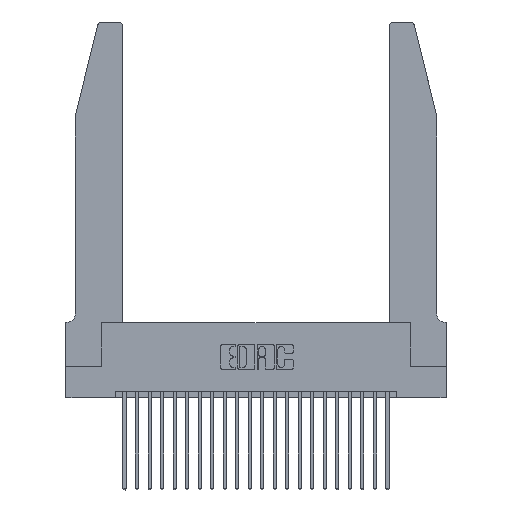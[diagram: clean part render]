
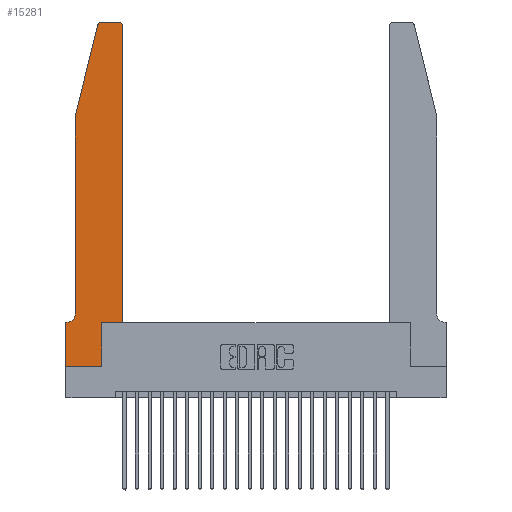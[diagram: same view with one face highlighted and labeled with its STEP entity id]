
A CAD part, top view. The second image highlights one B-rep face of the part: STEP entity #15281.
In plain terms, the highlighted planar face has unit normal (0, 0, 1).
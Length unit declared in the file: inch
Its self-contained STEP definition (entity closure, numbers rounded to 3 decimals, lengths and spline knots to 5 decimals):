
#43 = ORIENTED_EDGE ( 'NONE', *, *, #3046, .T. ) ;
#117 = VERTEX_POINT ( 'NONE', #5731 ) ;
#277 = ORIENTED_EDGE ( 'NONE', *, *, #18983, .T. ) ;
#382 = EDGE_LOOP ( 'NONE', ( #22888, #17297, #6636, #10401, #23073, #19586, #23817, #277, #12710, #6812, #18889, #43 ) ) ;
#537 = DIRECTION ( 'NONE',  ( 1., 0., 0. ) ) ;
#560 = LINE ( 'NONE', #15938, #16672 ) ;
#587 = EDGE_CURVE ( 'NONE', #2119, #10231, #1317, .T. ) ;
#693 = DIRECTION ( 'NONE',  ( 0., 0., 1. ) ) ;
#1015 = CARTESIAN_POINT ( 'NONE',  ( 0.0755, 2., 0.37 ) ) ;
#1059 = CARTESIAN_POINT ( 'NONE',  ( 0.0755, 0.42, 0.37 ) ) ;
#1317 = LINE ( 'NONE', #3193, #20154 ) ;
#1462 = VECTOR ( 'NONE', #9100, 39.37008 ) ;
#2029 = EDGE_CURVE ( 'NONE', #117, #14625, #18886, .T. ) ;
#2119 = VERTEX_POINT ( 'NONE', #3431 ) ;
#2405 = CARTESIAN_POINT ( 'NONE',  ( 0.284, 2.75, 0.37 ) ) ;
#2757 = CARTESIAN_POINT ( 'NONE',  ( 0., 0.35, 0.37 ) ) ;
#3012 = CARTESIAN_POINT ( 'NONE',  ( 0., 0., 0.37 ) ) ;
#3046 = EDGE_CURVE ( 'NONE', #17111, #22062, #6576, .T. ) ;
#3119 = VECTOR ( 'NONE', #14447, 39.37008 ) ;
#3193 = CARTESIAN_POINT ( 'NONE',  ( 0.0755, 0.35, 0.37 ) ) ;
#3431 = CARTESIAN_POINT ( 'NONE',  ( 0.0055, 0.35, 0.37 ) ) ;
#3630 = VERTEX_POINT ( 'NONE', #12774 ) ;
#3832 = CARTESIAN_POINT ( 'NONE',  ( 0.0055, 0.42, 0.37 ) ) ;
#3883 = CIRCLE ( 'NONE', #12302, 0.03 ) ;
#4542 = CARTESIAN_POINT ( 'NONE',  ( 0.284, 2.72, 0.37 ) ) ;
#4727 = VERTEX_POINT ( 'NONE', #1059 ) ;
#4865 = DIRECTION ( 'NONE',  ( -0.239, -0.971, 0. ) ) ;
#5518 = LINE ( 'NONE', #23951, #3119 ) ;
#5731 = CARTESIAN_POINT ( 'NONE',  ( 0.25487, 2.72718, 0.37 ) ) ;
#6071 = DIRECTION ( 'NONE',  ( 0., 0., 1. ) ) ;
#6576 = CIRCLE ( 'NONE', #12965, 0.03 ) ;
#6636 = ORIENTED_EDGE ( 'NONE', *, *, #2029, .T. ) ;
#6812 = ORIENTED_EDGE ( 'NONE', *, *, #21663, .T. ) ;
#7202 = CARTESIAN_POINT ( 'NONE',  ( 0.0755, 2., 0.37 ) ) ;
#7475 = EDGE_CURVE ( 'NONE', #14667, #3630, #17307, .T. ) ;
#7764 = CARTESIAN_POINT ( 'NONE',  ( 0.4505, 2.72, 0.37 ) ) ;
#9100 = DIRECTION ( 'NONE',  ( -1., 0., 0. ) ) ;
#10217 = DIRECTION ( 'NONE',  ( 1., 0., 0. ) ) ;
#10231 = VERTEX_POINT ( 'NONE', #2757 ) ;
#10401 = ORIENTED_EDGE ( 'NONE', *, *, #16230, .T. ) ;
#10717 = DIRECTION ( 'NONE',  ( 0., 0., 1. ) ) ;
#11966 = VECTOR ( 'NONE', #16384, 39.37008 ) ;
#11976 = CARTESIAN_POINT ( 'NONE',  ( 0.4205, 2.72, 0.37 ) ) ;
#12302 = AXIS2_PLACEMENT_3D ( 'NONE', #4542, #693, #17900 ) ;
#12348 = DIRECTION ( 'NONE',  ( 0., 1., 0. ) ) ;
#12536 = FACE_OUTER_BOUND ( 'NONE', #382, .T. ) ;
#12710 = ORIENTED_EDGE ( 'NONE', *, *, #7475, .T. ) ;
#12774 = CARTESIAN_POINT ( 'NONE',  ( 0.2865, 0.35, 0.37 ) ) ;
#12965 = AXIS2_PLACEMENT_3D ( 'NONE', #11976, #6071, #537 ) ;
#13073 = CARTESIAN_POINT ( 'NONE',  ( 0.2865, 0.35, 0.37 ) ) ;
#13374 = VECTOR ( 'NONE', #20413, 39.37008 ) ;
#13804 = CARTESIAN_POINT ( 'NONE',  ( 0.2605, 2.75, 0.37 ) ) ;
#14124 = EDGE_CURVE ( 'NONE', #19387, #117, #3883, .T. ) ;
#14238 = EDGE_CURVE ( 'NONE', #10231, #17722, #22120, .T. ) ;
#14254 = CIRCLE ( 'NONE', #17129, 0.07 ) ;
#14447 = DIRECTION ( 'NONE',  ( 1., 0., 0. ) ) ;
#14625 = VERTEX_POINT ( 'NONE', #23395 ) ;
#14667 = VERTEX_POINT ( 'NONE', #22562 ) ;
#15005 = VECTOR ( 'NONE', #4865, 39.37008 ) ;
#15069 = VECTOR ( 'NONE', #12348, 39.37008 ) ;
#15201 = AXIS2_PLACEMENT_3D ( 'NONE', #21933, #10717, #16190 ) ;
#15281 = ADVANCED_FACE ( 'NONE', ( #12536 ), #16506, .T. ) ;
#15475 = EDGE_CURVE ( 'NONE', #22062, #19387, #15828, .T. ) ;
#15488 = LINE ( 'NONE', #7202, #13374 ) ;
#15678 = LINE ( 'NONE', #18116, #15069 ) ;
#15800 = DIRECTION ( 'NONE',  ( -1., 0., 0. ) ) ;
#15828 = LINE ( 'NONE', #13804, #1462 ) ;
#15938 = CARTESIAN_POINT ( 'NONE',  ( 0., 0., 0.37 ) ) ;
#16128 = CARTESIAN_POINT ( 'NONE',  ( 0.4205, 2.75, 0.37 ) ) ;
#16190 = DIRECTION ( 'NONE',  ( 1., 0., 0. ) ) ;
#16230 = EDGE_CURVE ( 'NONE', #14625, #4727, #15488, .T. ) ;
#16384 = DIRECTION ( 'NONE',  ( 0., -1., 0. ) ) ;
#16506 = PLANE ( 'NONE',  #15201 ) ;
#16632 = EDGE_CURVE ( 'NONE', #4727, #2119, #14254, .T. ) ;
#16672 = VECTOR ( 'NONE', #10217, 39.37008 ) ;
#17111 = VERTEX_POINT ( 'NONE', #7764 ) ;
#17129 = AXIS2_PLACEMENT_3D ( 'NONE', #3832, #17199, #15800 ) ;
#17199 = DIRECTION ( 'NONE',  ( 0., 0., -1. ) ) ;
#17297 = ORIENTED_EDGE ( 'NONE', *, *, #14124, .T. ) ;
#17307 = LINE ( 'NONE', #13073, #24474 ) ;
#17722 = VERTEX_POINT ( 'NONE', #20531 ) ;
#17900 = DIRECTION ( 'NONE',  ( 1., 0., 0. ) ) ;
#18107 = VERTEX_POINT ( 'NONE', #18913 ) ;
#18116 = CARTESIAN_POINT ( 'NONE',  ( 0.4505, 0.35, 0.37 ) ) ;
#18409 = DIRECTION ( 'NONE',  ( -1., 0., 0. ) ) ;
#18886 = LINE ( 'NONE', #1015, #15005 ) ;
#18889 = ORIENTED_EDGE ( 'NONE', *, *, #22055, .T. ) ;
#18913 = CARTESIAN_POINT ( 'NONE',  ( 0.4505, 0.35, 0.37 ) ) ;
#18983 = EDGE_CURVE ( 'NONE', #17722, #14667, #560, .T. ) ;
#19387 = VERTEX_POINT ( 'NONE', #2405 ) ;
#19586 = ORIENTED_EDGE ( 'NONE', *, *, #587, .T. ) ;
#20154 = VECTOR ( 'NONE', #18409, 39.37008 ) ;
#20413 = DIRECTION ( 'NONE',  ( 0., -1., 0. ) ) ;
#20531 = CARTESIAN_POINT ( 'NONE',  ( 0., 0., 0.37 ) ) ;
#21166 = DIRECTION ( 'NONE',  ( 0., 1., 0. ) ) ;
#21663 = EDGE_CURVE ( 'NONE', #3630, #18107, #5518, .T. ) ;
#21933 = CARTESIAN_POINT ( 'NONE',  ( 0., 0.35, 0.37 ) ) ;
#22055 = EDGE_CURVE ( 'NONE', #18107, #17111, #15678, .T. ) ;
#22062 = VERTEX_POINT ( 'NONE', #16128 ) ;
#22120 = LINE ( 'NONE', #3012, #11966 ) ;
#22562 = CARTESIAN_POINT ( 'NONE',  ( 0.2865, 0., 0.37 ) ) ;
#22888 = ORIENTED_EDGE ( 'NONE', *, *, #15475, .T. ) ;
#23073 = ORIENTED_EDGE ( 'NONE', *, *, #16632, .T. ) ;
#23395 = CARTESIAN_POINT ( 'NONE',  ( 0.0755, 2., 0.37 ) ) ;
#23817 = ORIENTED_EDGE ( 'NONE', *, *, #14238, .T. ) ;
#23951 = CARTESIAN_POINT ( 'NONE',  ( 0.4505, 0.35, 0.37 ) ) ;
#24474 = VECTOR ( 'NONE', #21166, 39.37008 ) ;
